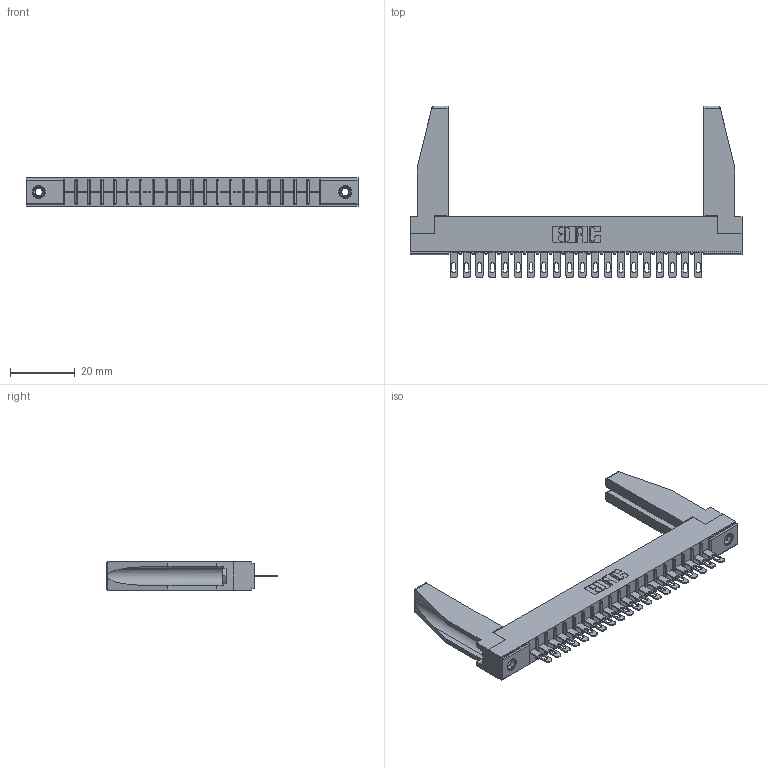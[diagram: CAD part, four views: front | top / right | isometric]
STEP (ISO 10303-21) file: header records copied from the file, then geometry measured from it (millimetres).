
FILE_DESCRIPTION (( 'STEP AP203' ), '1' );
FILE_NAME ('316-020-400-178.STEP', '2020-09-22T19:29:35', ( '' ), ( '' ), 'SwSTEP 2.0', 'SolidWorks 2020', '' );
FILE_SCHEMA (( 'CONFIG_CONTROL_DESIGN' ));
Length unit declared in the file: inch
Products named in the file (5): 307-220-078; 316-020-400-178; 306-290-001_100; 345-250-001_345-250-001-102; 306 Part_.156 Dia
Assembly tree (25 placements, depth 2):
  316-020-400-178
    306 Part_.156 Dia
    306-290-001_100  x20
    345-250-001_345-250-001-102  x2
    307-220-078  x2
Bounding box: 102.26 x 52.91 x 8.71 mm (x, y, z)
Volume: 11046.6 mm3; surface area: 14503.3 mm2
Topology: 25 solids, 25 shells, 1766 faces, 4946 edges, 3180 vertices
Faces by surface type: plane 1152, cylinder 518, sphere 80, cone 12, torus 4
Entity records: 24104 total; most frequent: CARTESIAN_POINT 4045, ORIENTED_EDGE 3966, DIRECTION 3943, EDGE_CURVE 1983, LINE 1539, VECTOR 1539, VERTEX_POINT 1262, AXIS2_PLACEMENT_3D 1202
